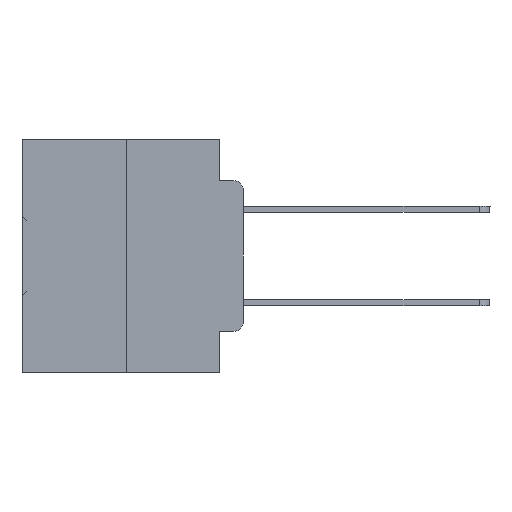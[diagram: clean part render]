
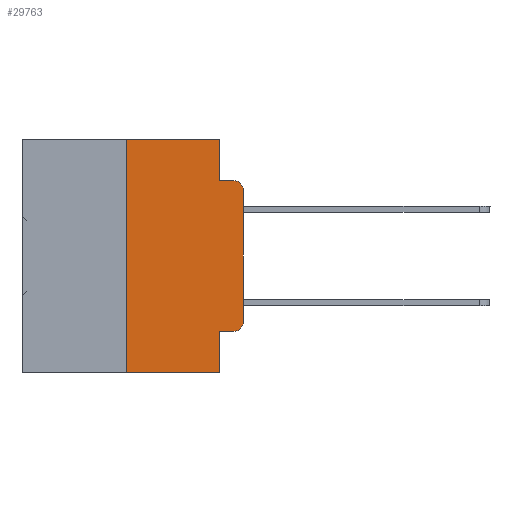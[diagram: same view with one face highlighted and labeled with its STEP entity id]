
A CAD part, left-side view. The second image highlights one B-rep face of the part: STEP entity #29763.
In plain terms, the highlighted planar face has unit normal (-1, 0, 0).
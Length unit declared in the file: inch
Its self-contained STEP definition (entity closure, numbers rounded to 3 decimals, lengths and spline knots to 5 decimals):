
#307 = DIRECTION ( 'NONE',  ( 0., -1., 0. ) ) ;
#407 = DIRECTION ( 'NONE',  ( 0., 0., -1. ) ) ;
#865 = VERTEX_POINT ( 'NONE', #5907 ) ;
#1028 = VECTOR ( 'NONE', #8561, 39.37008 ) ;
#1142 = VERTEX_POINT ( 'NONE', #36246 ) ;
#3027 = CARTESIAN_POINT ( 'NONE',  ( 0., 0.051, -0.0885 ) ) ;
#3374 = LINE ( 'NONE', #26173, #28084 ) ;
#3560 = CARTESIAN_POINT ( 'NONE',  ( 0., 0., -0.3915 ) ) ;
#3634 = ORIENTED_EDGE ( 'NONE', *, *, #19175, .T. ) ;
#4101 = VECTOR ( 'NONE', #34125, 39.37008 ) ;
#4128 = CARTESIAN_POINT ( 'NONE',  ( 0., 0.051, 0. ) ) ;
#4247 = EDGE_LOOP ( 'NONE', ( #27762, #3634, #34816, #5689, #22581, #34369, #24953, #25926, #27148, #26513 ) ) ;
#5581 = CARTESIAN_POINT ( 'NONE',  ( 0., 0.02, -0.3915 ) ) ;
#5689 = ORIENTED_EDGE ( 'NONE', *, *, #28378, .F. ) ;
#5907 = CARTESIAN_POINT ( 'NONE',  ( 0., 0.02, -0.4115 ) ) ;
#5948 = DIRECTION ( 'NONE',  ( 0., -1., 0. ) ) ;
#6080 = CIRCLE ( 'NONE', #21480, 0.02 ) ;
#6327 = EDGE_CURVE ( 'NONE', #23446, #22678, #9281, .T. ) ;
#6432 = CARTESIAN_POINT ( 'NONE',  ( 0., 0.25, -0.5 ) ) ;
#7107 = VERTEX_POINT ( 'NONE', #6432 ) ;
#7684 = CARTESIAN_POINT ( 'NONE',  ( 0., 0.051, -0.4115 ) ) ;
#7992 = DIRECTION ( 'NONE',  ( 0., 0., -1. ) ) ;
#8561 = DIRECTION ( 'NONE',  ( 0., -1., 0. ) ) ;
#8954 = AXIS2_PLACEMENT_3D ( 'NONE', #9293, #19897, #23032 ) ;
#9106 = EDGE_CURVE ( 'NONE', #35510, #13974, #18244, .T. ) ;
#9179 = CARTESIAN_POINT ( 'NONE',  ( 0., 0.02, -0.1085 ) ) ;
#9281 = LINE ( 'NONE', #3027, #4101 ) ;
#9293 = CARTESIAN_POINT ( 'NONE',  ( 0., 0.473, 0. ) ) ;
#9394 = EDGE_CURVE ( 'NONE', #17955, #865, #33947, .T. ) ;
#11683 = LINE ( 'NONE', #23170, #22491 ) ;
#11904 = PLANE ( 'NONE',  #8954 ) ;
#12044 = AXIS2_PLACEMENT_3D ( 'NONE', #9179, #20503, #20858 ) ;
#13974 = VERTEX_POINT ( 'NONE', #17754 ) ;
#14146 = CARTESIAN_POINT ( 'NONE',  ( 0., 0.051, -0.4115 ) ) ;
#15705 = EDGE_CURVE ( 'NONE', #1142, #18472, #16987, .T. ) ;
#16861 = EDGE_CURVE ( 'NONE', #7107, #36107, #25788, .T. ) ;
#16987 = LINE ( 'NONE', #31224, #29091 ) ;
#17754 = CARTESIAN_POINT ( 'NONE',  ( 0., 0., -0.1085 ) ) ;
#17955 = VERTEX_POINT ( 'NONE', #7684 ) ;
#18244 = LINE ( 'NONE', #32672, #28207 ) ;
#18472 = VERTEX_POINT ( 'NONE', #4128 ) ;
#18678 = CARTESIAN_POINT ( 'NONE',  ( 0., 0.051, 0. ) ) ;
#19175 = EDGE_CURVE ( 'NONE', #13974, #22678, #33352, .T. ) ;
#19310 = CARTESIAN_POINT ( 'NONE',  ( 0., 0.051, -0.0885 ) ) ;
#19897 = DIRECTION ( 'NONE',  ( 1., 0., 0. ) ) ;
#19945 = CARTESIAN_POINT ( 'NONE',  ( 0., 0.02, -0.0885 ) ) ;
#20255 = FACE_OUTER_BOUND ( 'NONE', #4247, .T. ) ;
#20503 = DIRECTION ( 'NONE',  ( -1., 0., 0. ) ) ;
#20858 = DIRECTION ( 'NONE',  ( 0., 0., -1. ) ) ;
#21077 = DIRECTION ( 'NONE',  ( 0., 0., -1. ) ) ;
#21480 = AXIS2_PLACEMENT_3D ( 'NONE', #5581, #25067, #7992 ) ;
#22491 = VECTOR ( 'NONE', #407, 39.37008 ) ;
#22581 = ORIENTED_EDGE ( 'NONE', *, *, #15705, .F. ) ;
#22678 = VERTEX_POINT ( 'NONE', #19945 ) ;
#23032 = DIRECTION ( 'NONE',  ( 0., 0., -1. ) ) ;
#23170 = CARTESIAN_POINT ( 'NONE',  ( 0., 0.051, 0. ) ) ;
#23446 = VERTEX_POINT ( 'NONE', #19310 ) ;
#24953 = ORIENTED_EDGE ( 'NONE', *, *, #16861, .T. ) ;
#25067 = DIRECTION ( 'NONE',  ( -1., 0., 0. ) ) ;
#25788 = LINE ( 'NONE', #28193, #30368 ) ;
#25926 = ORIENTED_EDGE ( 'NONE', *, *, #27745, .F. ) ;
#26173 = CARTESIAN_POINT ( 'NONE',  ( 0., 0.25, 0. ) ) ;
#26513 = ORIENTED_EDGE ( 'NONE', *, *, #33294, .T. ) ;
#27148 = ORIENTED_EDGE ( 'NONE', *, *, #9394, .T. ) ;
#27745 = EDGE_CURVE ( 'NONE', #17955, #36107, #11683, .T. ) ;
#27762 = ORIENTED_EDGE ( 'NONE', *, *, #9106, .T. ) ;
#28084 = VECTOR ( 'NONE', #28400, 39.37008 ) ;
#28193 = CARTESIAN_POINT ( 'NONE',  ( 0., 0.473, -0.5 ) ) ;
#28207 = VECTOR ( 'NONE', #29535, 39.37008 ) ;
#28378 = EDGE_CURVE ( 'NONE', #18472, #23446, #35517, .T. ) ;
#28400 = DIRECTION ( 'NONE',  ( 0., 0., 1. ) ) ;
#29091 = VECTOR ( 'NONE', #307, 39.37008 ) ;
#29535 = DIRECTION ( 'NONE',  ( 0., 0., 1. ) ) ;
#29763 = ADVANCED_FACE ( 'NONE', ( #20255 ), #11904, .F. ) ;
#30368 = VECTOR ( 'NONE', #5948, 39.37008 ) ;
#30782 = VECTOR ( 'NONE', #21077, 39.37008 ) ;
#31224 = CARTESIAN_POINT ( 'NONE',  ( 0., 0.473, 0. ) ) ;
#32672 = CARTESIAN_POINT ( 'NONE',  ( 0., 0., 0. ) ) ;
#33294 = EDGE_CURVE ( 'NONE', #865, #35510, #6080, .T. ) ;
#33352 = CIRCLE ( 'NONE', #12044, 0.02 ) ;
#33947 = LINE ( 'NONE', #14146, #1028 ) ;
#34125 = DIRECTION ( 'NONE',  ( 0., -1., 0. ) ) ;
#34369 = ORIENTED_EDGE ( 'NONE', *, *, #35397, .F. ) ;
#34816 = ORIENTED_EDGE ( 'NONE', *, *, #6327, .F. ) ;
#35397 = EDGE_CURVE ( 'NONE', #7107, #1142, #3374, .T. ) ;
#35510 = VERTEX_POINT ( 'NONE', #3560 ) ;
#35517 = LINE ( 'NONE', #18678, #30782 ) ;
#35906 = CARTESIAN_POINT ( 'NONE',  ( 0., 0.051, -0.5 ) ) ;
#36107 = VERTEX_POINT ( 'NONE', #35906 ) ;
#36246 = CARTESIAN_POINT ( 'NONE',  ( 0., 0.25, 0. ) ) ;
